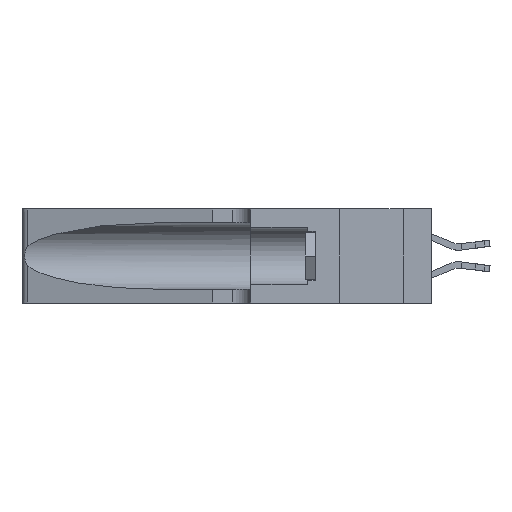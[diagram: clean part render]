
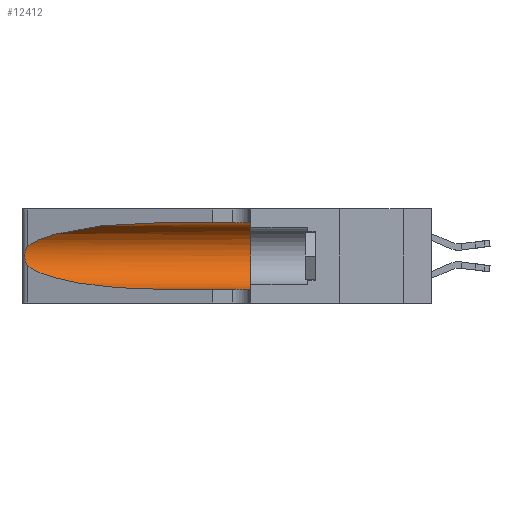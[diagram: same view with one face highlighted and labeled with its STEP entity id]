
A CAD part, left-side view. The second image highlights one B-rep face of the part: STEP entity #12412.
In plain terms, the highlighted cylindrical face has radius 3.308 mm (diameter 6.617 mm), a partial arc.
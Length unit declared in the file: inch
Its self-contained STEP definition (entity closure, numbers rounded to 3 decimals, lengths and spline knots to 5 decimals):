
#63 = VERTEX_POINT ( 'NONE', #12691 ) ;
#411 = CARTESIAN_POINT ( 'NONE',  ( 0.25487, 1.22718, 0.14631 ) ) ;
#529 = EDGE_CURVE ( 'NONE', #2132, #14018, #12624, .T. ) ;
#1216 = VERTEX_POINT ( 'NONE', #13309 ) ;
#1732 = CARTESIAN_POINT ( 'NONE',  ( 0.1305, 0.35, 0.185 ) ) ;
#1828 = LINE ( 'NONE', #7522, #23976 ) ;
#2132 = VERTEX_POINT ( 'NONE', #27419 ) ;
#2807 = CARTESIAN_POINT ( 'NONE',  ( 0.1305, 0.72297, 0.05475 ) ) ;
#2904 = CARTESIAN_POINT ( 'NONE',  ( 0.2373, 1.15595, 0.08982 ) ) ;
#3380 = ORIENTED_EDGE ( 'NONE', *, *, #529, .F. ) ;
#3566 = CARTESIAN_POINT ( 'NONE',  ( 0.25789, 1.23486, 0.15765 ) ) ;
#3775 = FACE_OUTER_BOUND ( 'NONE', #22021, .T. ) ;
#4418 = CARTESIAN_POINT ( 'NONE',  ( 0.1305, 0.72297, 0.31525 ) ) ;
#4608 = CARTESIAN_POINT ( 'NONE',  ( 0.1305, 0.72297, 0.31525 ) ) ;
#4809 = CARTESIAN_POINT ( 'NONE',  ( 0.18966, 0.96281, 0.05475 ) ) ;
#5317 = EDGE_CURVE ( 'NONE', #7241, #23784, #26733, .T. ) ;
#5558 = CARTESIAN_POINT ( 'NONE',  ( 0.25854, 1.2359, 0.20912 ) ) ;
#6720 = ORIENTED_EDGE ( 'NONE', *, *, #10604, .F. ) ;
#7062 = CARTESIAN_POINT ( 'NONE',  ( 0.1305, 1.61858, 0.31525 ) ) ;
#7137 = AXIS2_PLACEMENT_3D ( 'NONE', #11227, #15459, #17516 ) ;
#7241 = VERTEX_POINT ( 'NONE', #4608 ) ;
#7522 = CARTESIAN_POINT ( 'NONE',  ( 0.1305, 1.61858, 0.05475 ) ) ;
#7926 = CARTESIAN_POINT ( 'NONE',  ( 0.25555, 1.22993, 0.14849 ) ) ;
#8214 = B_SPLINE_CURVE_WITH_KNOTS ( 'NONE', 3,
 ( #20961, #9861, #16416, #12214, #5558, #22981, #22591, #10140, #24746, #27169, #3566, #25114, #7926, #11932 ),
 .UNSPECIFIED., .F., .F.,
 ( 4, 2, 2, 2, 2, 2, 4 ),
 ( 0., 0.00027, 0.00053, 0.00107, 0.0016, 0.00187, 0.00214 ),
 .UNSPECIFIED. ) ;
#8690 = CARTESIAN_POINT ( 'NONE',  ( 0.18966, 0.96281, 0.31525 ) ) ;
#8892 = EDGE_CURVE ( 'NONE', #23784, #1216, #8214, .T. ) ;
#9861 = CARTESIAN_POINT ( 'NONE',  ( 0.25555, 1.22994, 0.2215 ) ) ;
#10140 = CARTESIAN_POINT ( 'NONE',  ( 0.26075, 1.23896, 0.178 ) ) ;
#10402 = EDGE_CURVE ( 'NONE', #63, #14018, #1828, .T. ) ;
#10417 = DIRECTION ( 'NONE',  ( 0., 1., 0. ) ) ;
#10453 = CARTESIAN_POINT ( 'NONE',  ( 0.25487, 1.22718, 0.22369 ) ) ;
#10604 = EDGE_CURVE ( 'NONE', #7241, #2132, #17611, .T. ) ;
#11227 = CARTESIAN_POINT ( 'NONE',  ( 0.1305, 1.61858, 0.185 ) ) ;
#11932 = CARTESIAN_POINT ( 'NONE',  ( 0.25487, 1.22718, 0.14631 ) ) ;
#12214 = CARTESIAN_POINT ( 'NONE',  ( 0.25787, 1.23484, 0.2124 ) ) ;
#12290 = DIRECTION ( 'NONE',  ( 0., -1., 0. ) ) ;
#12412 = ADVANCED_FACE ( 'NONE', ( #3775 ), #12540, .F. ) ;
#12540 = CYLINDRICAL_SURFACE ( 'NONE', #7137, 0.13025 ) ;
#12624 = CIRCLE ( 'NONE', #21452, 0.13025 ) ;
#12691 = CARTESIAN_POINT ( 'NONE',  ( 0.1305, 0.72297, 0.05475 ) ) ;
#13309 = CARTESIAN_POINT ( 'NONE',  ( 0.25487, 1.22718, 0.14631 ) ) ;
#13680 =( BOUNDED_CURVE ( )  B_SPLINE_CURVE ( 3, ( #411, #2904, #4809, #2807 ),
 .UNSPECIFIED., .F., .T. ) 
 B_SPLINE_CURVE_WITH_KNOTS ( ( 4, 4 ),
 ( 3.44316, 4.71239 ),
 .UNSPECIFIED. ) 
 CURVE ( )  GEOMETRIC_REPRESENTATION_ITEM ( )  RATIONAL_B_SPLINE_CURVE ( ( 1., 0.87, 0.87, 1. ) ) 
 REPRESENTATION_ITEM ( '' )  );
#14018 = VERTEX_POINT ( 'NONE', #18758 ) ;
#15057 = CARTESIAN_POINT ( 'NONE',  ( 0.2373, 1.15595, 0.28018 ) ) ;
#15459 = DIRECTION ( 'NONE',  ( 0., -1., 0. ) ) ;
#16416 = CARTESIAN_POINT ( 'NONE',  ( 0.25639, 1.23184, 0.21858 ) ) ;
#17301 = VECTOR ( 'NONE', #18413, 39.37008 ) ;
#17516 = DIRECTION ( 'NONE',  ( 0., 0., -1. ) ) ;
#17611 = LINE ( 'NONE', #7062, #17301 ) ;
#18389 = ORIENTED_EDGE ( 'NONE', *, *, #8892, .T. ) ;
#18413 = DIRECTION ( 'NONE',  ( 0., -1., 0. ) ) ;
#18758 = CARTESIAN_POINT ( 'NONE',  ( 0.1305, 0.35, 0.05475 ) ) ;
#18776 = ORIENTED_EDGE ( 'NONE', *, *, #10402, .T. ) ;
#19648 = CARTESIAN_POINT ( 'NONE',  ( 0.25487, 1.22718, 0.22369 ) ) ;
#20648 = ORIENTED_EDGE ( 'NONE', *, *, #24057, .T. ) ;
#20961 = CARTESIAN_POINT ( 'NONE',  ( 0.25487, 1.22718, 0.22369 ) ) ;
#21040 = DIRECTION ( 'NONE',  ( 0., 0., 1. ) ) ;
#21452 = AXIS2_PLACEMENT_3D ( 'NONE', #1732, #10417, #21040 ) ;
#22021 = EDGE_LOOP ( 'NONE', ( #26842, #18389, #20648, #18776, #3380, #6720 ) ) ;
#22591 = CARTESIAN_POINT ( 'NONE',  ( 0.26075, 1.23896, 0.19203 ) ) ;
#22981 = CARTESIAN_POINT ( 'NONE',  ( 0.26018, 1.23835, 0.19895 ) ) ;
#23784 = VERTEX_POINT ( 'NONE', #10453 ) ;
#23976 = VECTOR ( 'NONE', #12290, 39.37008 ) ;
#24057 = EDGE_CURVE ( 'NONE', #1216, #63, #13680, .T. ) ;
#24746 = CARTESIAN_POINT ( 'NONE',  ( 0.26017, 1.23833, 0.17102 ) ) ;
#25114 = CARTESIAN_POINT ( 'NONE',  ( 0.25639, 1.23186, 0.15144 ) ) ;
#26733 =( BOUNDED_CURVE ( )  B_SPLINE_CURVE ( 3, ( #4418, #8690, #15057, #19648 ),
 .UNSPECIFIED., .F., .F. ) 
 B_SPLINE_CURVE_WITH_KNOTS ( ( 4, 4 ),
 ( 1.5708, 2.84003 ),
 .UNSPECIFIED. ) 
 CURVE ( )  GEOMETRIC_REPRESENTATION_ITEM ( )  RATIONAL_B_SPLINE_CURVE ( ( 1., 0.87, 0.87, 1. ) ) 
 REPRESENTATION_ITEM ( '' )  );
#26842 = ORIENTED_EDGE ( 'NONE', *, *, #5317, .T. ) ;
#27169 = CARTESIAN_POINT ( 'NONE',  ( 0.25856, 1.23593, 0.16098 ) ) ;
#27419 = CARTESIAN_POINT ( 'NONE',  ( 0.1305, 0.35, 0.31525 ) ) ;
